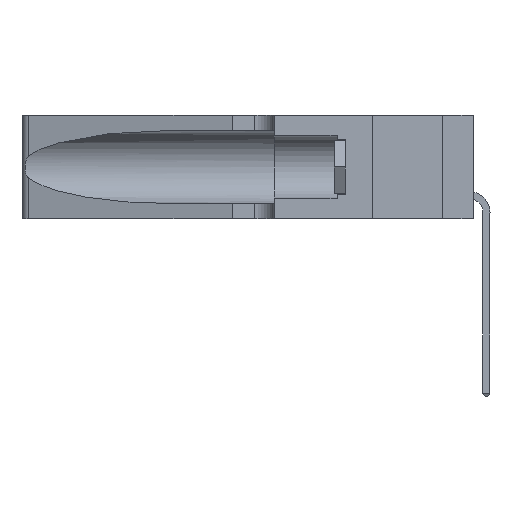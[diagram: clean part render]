
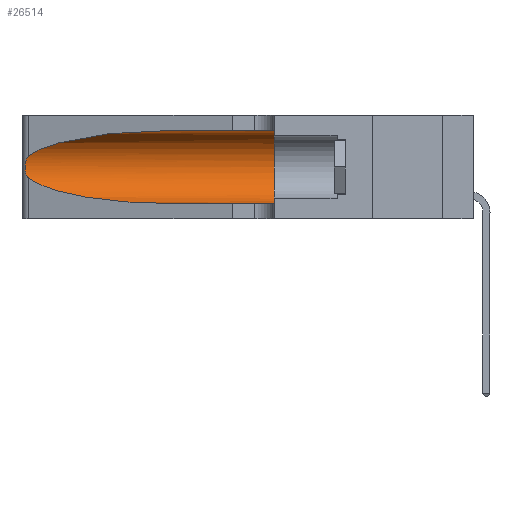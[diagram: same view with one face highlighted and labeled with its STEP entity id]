
A CAD part, left-side view. The second image highlights one B-rep face of the part: STEP entity #26514.
In plain terms, the highlighted cylindrical face has radius 3.308 mm (diameter 6.617 mm), a partial arc.
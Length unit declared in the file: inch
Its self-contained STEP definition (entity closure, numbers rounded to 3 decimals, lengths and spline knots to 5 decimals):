
#1744 =( BOUNDED_CURVE ( )  B_SPLINE_CURVE ( 3, ( #36429, #29940, #2328, #21382 ),
 .UNSPECIFIED., .F., .F. ) 
 B_SPLINE_CURVE_WITH_KNOTS ( ( 4, 4 ),
 ( 3.44316, 4.71239 ),
 .UNSPECIFIED. ) 
 CURVE ( )  GEOMETRIC_REPRESENTATION_ITEM ( )  RATIONAL_B_SPLINE_CURVE ( ( 1., 0.87, 0.87, 1. ) ) 
 REPRESENTATION_ITEM ( '' )  );
#2046 = LINE ( 'NONE', #17663, #32566 ) ;
#2328 = CARTESIAN_POINT ( 'NONE',  ( 0.18966, 0.96281, 0.05475 ) ) ;
#2347 = CYLINDRICAL_SURFACE ( 'NONE', #3458, 0.13025 ) ;
#3458 = AXIS2_PLACEMENT_3D ( 'NONE', #10531, #13661, #23298 ) ;
#3671 = DIRECTION ( 'NONE',  ( 0., 1., 0. ) ) ;
#3724 = EDGE_CURVE ( 'NONE', #9975, #39978, #1744, .T. ) ;
#3925 = CARTESIAN_POINT ( 'NONE',  ( 0.26075, 1.23896, 0.178 ) ) ;
#4060 = CARTESIAN_POINT ( 'NONE',  ( 0.25555, 1.22994, 0.2215 ) ) ;
#5880 = CIRCLE ( 'NONE', #12125, 0.13025 ) ;
#5943 = EDGE_CURVE ( 'NONE', #34252, #24271, #5880, .T. ) ;
#6408 = CARTESIAN_POINT ( 'NONE',  ( 0.1305, 0.35, 0.05475 ) ) ;
#6520 = CARTESIAN_POINT ( 'NONE',  ( 0.26018, 1.23835, 0.19895 ) ) ;
#6608 = LINE ( 'NONE', #16283, #12388 ) ;
#6659 = CARTESIAN_POINT ( 'NONE',  ( 0.25487, 1.22718, 0.22369 ) ) ;
#6753 = VERTEX_POINT ( 'NONE', #23263 ) ;
#8398 = ORIENTED_EDGE ( 'NONE', *, *, #34906, .T. ) ;
#9885 = DIRECTION ( 'NONE',  ( 0., 0., 1. ) ) ;
#9975 = VERTEX_POINT ( 'NONE', #11093 ) ;
#10531 = CARTESIAN_POINT ( 'NONE',  ( 0.1305, 1.61858, 0.185 ) ) ;
#11093 = CARTESIAN_POINT ( 'NONE',  ( 0.25487, 1.22718, 0.14631 ) ) ;
#11277 = DIRECTION ( 'NONE',  ( 0., -1., 0. ) ) ;
#12125 = AXIS2_PLACEMENT_3D ( 'NONE', #19093, #3671, #9885 ) ;
#12246 = ORIENTED_EDGE ( 'NONE', *, *, #5943, .F. ) ;
#12388 = VECTOR ( 'NONE', #28726, 39.37008 ) ;
#12882 = CARTESIAN_POINT ( 'NONE',  ( 0.25555, 1.22993, 0.14849 ) ) ;
#12953 = ORIENTED_EDGE ( 'NONE', *, *, #27414, .F. ) ;
#13140 = CARTESIAN_POINT ( 'NONE',  ( 0.2373, 1.15595, 0.28018 ) ) ;
#13661 = DIRECTION ( 'NONE',  ( 0., -1., 0. ) ) ;
#15640 = CARTESIAN_POINT ( 'NONE',  ( 0.1305, 0.35, 0.31525 ) ) ;
#16283 = CARTESIAN_POINT ( 'NONE',  ( 0.1305, 1.61858, 0.05475 ) ) ;
#16284 = CARTESIAN_POINT ( 'NONE',  ( 0.25487, 1.22718, 0.22369 ) ) ;
#16384 = EDGE_LOOP ( 'NONE', ( #8398, #16638, #38719, #27192, #12246, #12953 ) ) ;
#16419 = CARTESIAN_POINT ( 'NONE',  ( 0.25787, 1.23484, 0.2124 ) ) ;
#16638 = ORIENTED_EDGE ( 'NONE', *, *, #28213, .T. ) ;
#16716 = EDGE_CURVE ( 'NONE', #39978, #24271, #6608, .T. ) ;
#16881 =( BOUNDED_CURVE ( )  B_SPLINE_CURVE ( 3, ( #34684, #31686, #13140, #6659 ),
 .UNSPECIFIED., .F., .T. ) 
 B_SPLINE_CURVE_WITH_KNOTS ( ( 4, 4 ),
 ( 1.5708, 2.84003 ),
 .UNSPECIFIED. ) 
 CURVE ( )  GEOMETRIC_REPRESENTATION_ITEM ( )  RATIONAL_B_SPLINE_CURVE ( ( 1., 0.87, 0.87, 1. ) ) 
 REPRESENTATION_ITEM ( '' )  );
#17663 = CARTESIAN_POINT ( 'NONE',  ( 0.1305, 1.61858, 0.31525 ) ) ;
#18977 = CARTESIAN_POINT ( 'NONE',  ( 0.25789, 1.23486, 0.15765 ) ) ;
#19093 = CARTESIAN_POINT ( 'NONE',  ( 0.1305, 0.35, 0.185 ) ) ;
#21382 = CARTESIAN_POINT ( 'NONE',  ( 0.1305, 0.72297, 0.05475 ) ) ;
#22100 = CARTESIAN_POINT ( 'NONE',  ( 0.25639, 1.23186, 0.15144 ) ) ;
#22509 = CARTESIAN_POINT ( 'NONE',  ( 0.25854, 1.2359, 0.20912 ) ) ;
#22748 = CARTESIAN_POINT ( 'NONE',  ( 0.1305, 0.72297, 0.31525 ) ) ;
#23263 = CARTESIAN_POINT ( 'NONE',  ( 0.25487, 1.22718, 0.22369 ) ) ;
#23298 = DIRECTION ( 'NONE',  ( 0., 0., -1. ) ) ;
#24271 = VERTEX_POINT ( 'NONE', #6408 ) ;
#25165 = VERTEX_POINT ( 'NONE', #22748 ) ;
#25627 = CARTESIAN_POINT ( 'NONE',  ( 0.25856, 1.23593, 0.16098 ) ) ;
#26514 = ADVANCED_FACE ( 'NONE', ( #30405 ), #2347, .F. ) ;
#27042 = B_SPLINE_CURVE_WITH_KNOTS ( 'NONE', 3,
 ( #16284, #4060, #34544, #16419, #22509, #6520, #28188, #3925, #31292, #25627, #18977, #22100, #12882, #37709 ),
 .UNSPECIFIED., .F., .F.,
 ( 4, 2, 2, 2, 2, 2, 4 ),
 ( 0., 0.00027, 0.00053, 0.00107, 0.0016, 0.00187, 0.00214 ),
 .UNSPECIFIED. ) ;
#27192 = ORIENTED_EDGE ( 'NONE', *, *, #16716, .T. ) ;
#27414 = EDGE_CURVE ( 'NONE', #25165, #34252, #2046, .T. ) ;
#28188 = CARTESIAN_POINT ( 'NONE',  ( 0.26075, 1.23896, 0.19203 ) ) ;
#28213 = EDGE_CURVE ( 'NONE', #6753, #9975, #27042, .T. ) ;
#28726 = DIRECTION ( 'NONE',  ( 0., -1., 0. ) ) ;
#29940 = CARTESIAN_POINT ( 'NONE',  ( 0.2373, 1.15595, 0.08982 ) ) ;
#30405 = FACE_OUTER_BOUND ( 'NONE', #16384, .T. ) ;
#31292 = CARTESIAN_POINT ( 'NONE',  ( 0.26017, 1.23833, 0.17102 ) ) ;
#31488 = CARTESIAN_POINT ( 'NONE',  ( 0.1305, 0.72297, 0.05475 ) ) ;
#31686 = CARTESIAN_POINT ( 'NONE',  ( 0.18966, 0.96281, 0.31525 ) ) ;
#32566 = VECTOR ( 'NONE', #11277, 39.37008 ) ;
#34252 = VERTEX_POINT ( 'NONE', #15640 ) ;
#34544 = CARTESIAN_POINT ( 'NONE',  ( 0.25639, 1.23184, 0.21858 ) ) ;
#34684 = CARTESIAN_POINT ( 'NONE',  ( 0.1305, 0.72297, 0.31525 ) ) ;
#34906 = EDGE_CURVE ( 'NONE', #25165, #6753, #16881, .T. ) ;
#36429 = CARTESIAN_POINT ( 'NONE',  ( 0.25487, 1.22718, 0.14631 ) ) ;
#37709 = CARTESIAN_POINT ( 'NONE',  ( 0.25487, 1.22718, 0.14631 ) ) ;
#38719 = ORIENTED_EDGE ( 'NONE', *, *, #3724, .T. ) ;
#39978 = VERTEX_POINT ( 'NONE', #31488 ) ;
